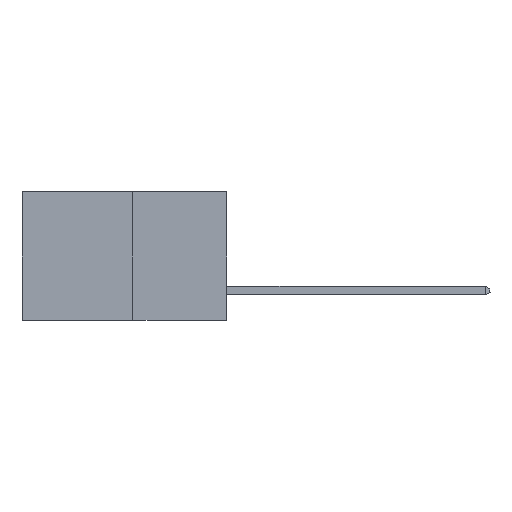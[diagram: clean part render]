
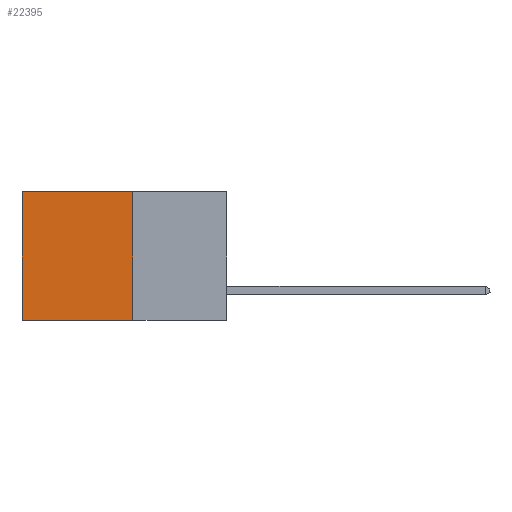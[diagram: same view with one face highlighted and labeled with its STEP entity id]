
A CAD part, left-side view. The second image highlights one B-rep face of the part: STEP entity #22395.
In plain terms, the highlighted planar face has unit normal (-1, 0, 0).
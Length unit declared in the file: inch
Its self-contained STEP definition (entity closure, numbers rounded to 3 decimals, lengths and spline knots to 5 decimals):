
#1003 = FACE_OUTER_BOUND ( 'NONE', #24845, .T. ) ;
#1664 = LINE ( 'NONE', #8003, #23531 ) ;
#2115 = PLANE ( 'NONE',  #11318 ) ;
#2263 = LINE ( 'NONE', #10517, #18546 ) ;
#2528 = CARTESIAN_POINT ( 'NONE',  ( 0.277, 0.27, -0.37 ) ) ;
#6320 = CARTESIAN_POINT ( 'NONE',  ( 0.277, 0.27, 0. ) ) ;
#6555 = VERTEX_POINT ( 'NONE', #6320 ) ;
#6816 = LINE ( 'NONE', #16988, #17468 ) ;
#8003 = CARTESIAN_POINT ( 'NONE',  ( 0.277, 0.59, -0.37 ) ) ;
#8514 = DIRECTION ( 'NONE',  ( 1., 0., 0. ) ) ;
#10517 = CARTESIAN_POINT ( 'NONE',  ( 0.277, 0.27, 0. ) ) ;
#11318 = AXIS2_PLACEMENT_3D ( 'NONE', #21241, #8514, #23318 ) ;
#11921 = LINE ( 'NONE', #2528, #23189 ) ;
#12245 = VERTEX_POINT ( 'NONE', #24328 ) ;
#12670 = DIRECTION ( 'NONE',  ( 0., 1., 0. ) ) ;
#14168 = EDGE_CURVE ( 'NONE', #24862, #12245, #1664, .T. ) ;
#14456 = EDGE_CURVE ( 'NONE', #6555, #23871, #11921, .T. ) ;
#15446 = EDGE_CURVE ( 'NONE', #6555, #24862, #2263, .T. ) ;
#16988 = CARTESIAN_POINT ( 'NONE',  ( 0.277, 0.27, -0.37 ) ) ;
#17118 = CARTESIAN_POINT ( 'NONE',  ( 0.277, 0.27, -0.37 ) ) ;
#17468 = VECTOR ( 'NONE', #19108, 39.37008 ) ;
#17699 = EDGE_CURVE ( 'NONE', #23871, #12245, #6816, .T. ) ;
#18097 = CARTESIAN_POINT ( 'NONE',  ( 0.277, 0.59, 0. ) ) ;
#18546 = VECTOR ( 'NONE', #12670, 39.37008 ) ;
#19108 = DIRECTION ( 'NONE',  ( 0., 1., 0. ) ) ;
#19996 = ORIENTED_EDGE ( 'NONE', *, *, #15446, .T. ) ;
#21241 = CARTESIAN_POINT ( 'NONE',  ( 0.277, 0.27, -0.37 ) ) ;
#21638 = DIRECTION ( 'NONE',  ( 0., 0., -1. ) ) ;
#22205 = ORIENTED_EDGE ( 'NONE', *, *, #14168, .T. ) ;
#22395 = ADVANCED_FACE ( 'NONE', ( #1003 ), #2115, .F. ) ;
#23189 = VECTOR ( 'NONE', #21638, 39.37008 ) ;
#23318 = DIRECTION ( 'NONE',  ( 0., 0., -1. ) ) ;
#23531 = VECTOR ( 'NONE', #26869, 39.37008 ) ;
#23871 = VERTEX_POINT ( 'NONE', #17118 ) ;
#24328 = CARTESIAN_POINT ( 'NONE',  ( 0.277, 0.59, -0.37 ) ) ;
#24845 = EDGE_LOOP ( 'NONE', ( #22205, #25502, #27112, #19996 ) ) ;
#24862 = VERTEX_POINT ( 'NONE', #18097 ) ;
#25502 = ORIENTED_EDGE ( 'NONE', *, *, #17699, .F. ) ;
#26869 = DIRECTION ( 'NONE',  ( 0., 0., -1. ) ) ;
#27112 = ORIENTED_EDGE ( 'NONE', *, *, #14456, .F. ) ;
